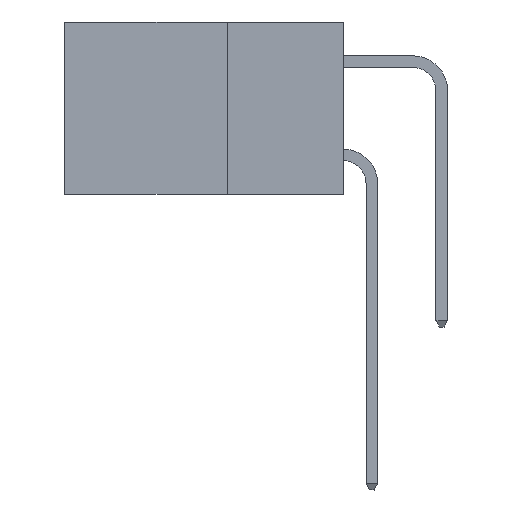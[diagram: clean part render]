
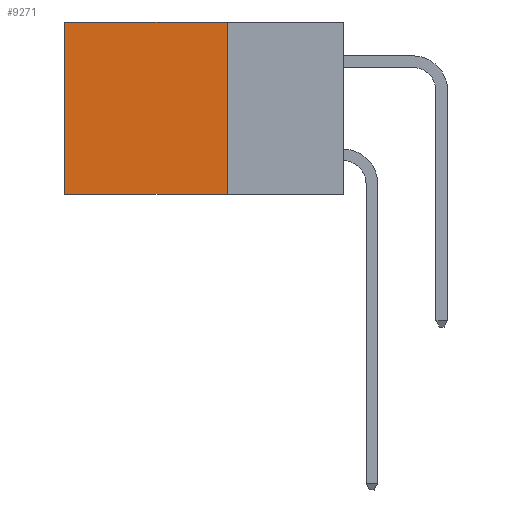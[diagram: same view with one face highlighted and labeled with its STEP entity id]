
A CAD part, left-side view. The second image highlights one B-rep face of the part: STEP entity #9271.
In plain terms, the highlighted planar face has unit normal (-1, 0, 0).
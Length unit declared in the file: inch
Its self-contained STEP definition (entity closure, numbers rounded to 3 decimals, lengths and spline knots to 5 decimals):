
#986 = FACE_OUTER_BOUND ( 'NONE', #16555, .T. ) ;
#1271 = CARTESIAN_POINT ( 'NONE',  ( 0.298, 0.25, -0.37 ) ) ;
#1565 = EDGE_CURVE ( 'NONE', #10299, #5157, #3699, .T. ) ;
#3554 = ORIENTED_EDGE ( 'NONE', *, *, #6476, .F. ) ;
#3699 = LINE ( 'NONE', #14299, #8437 ) ;
#5137 = EDGE_CURVE ( 'NONE', #11124, #12029, #8122, .T. ) ;
#5157 = VERTEX_POINT ( 'NONE', #9886 ) ;
#5939 = DIRECTION ( 'NONE',  ( 0., 0., -1. ) ) ;
#6021 = LINE ( 'NONE', #1271, #13595 ) ;
#6247 = DIRECTION ( 'NONE',  ( 0., 1., 0. ) ) ;
#6289 = VECTOR ( 'NONE', #13048, 39.37008 ) ;
#6476 = EDGE_CURVE ( 'NONE', #12029, #5157, #6021, .T. ) ;
#8122 = LINE ( 'NONE', #13840, #12003 ) ;
#8437 = VECTOR ( 'NONE', #16834, 39.37008 ) ;
#9271 = ADVANCED_FACE ( 'NONE', ( #986 ), #14039, .F. ) ;
#9448 = EDGE_CURVE ( 'NONE', #11124, #10299, #10170, .T. ) ;
#9886 = CARTESIAN_POINT ( 'NONE',  ( 0.298, 0.6, -0.37 ) ) ;
#10089 = CARTESIAN_POINT ( 'NONE',  ( 0.298, 0.25, 0. ) ) ;
#10170 = LINE ( 'NONE', #12938, #6289 ) ;
#10246 = DIRECTION ( 'NONE',  ( 0., 0., -1. ) ) ;
#10299 = VERTEX_POINT ( 'NONE', #11484 ) ;
#10909 = CARTESIAN_POINT ( 'NONE',  ( 0.298, 0.25, -0.37 ) ) ;
#11057 = CARTESIAN_POINT ( 'NONE',  ( 0.298, 0.25, 0. ) ) ;
#11124 = VERTEX_POINT ( 'NONE', #11057 ) ;
#11484 = CARTESIAN_POINT ( 'NONE',  ( 0.298, 0.6, 0. ) ) ;
#11871 = AXIS2_PLACEMENT_3D ( 'NONE', #10089, #13986, #10246 ) ;
#12003 = VECTOR ( 'NONE', #5939, 39.37008 ) ;
#12029 = VERTEX_POINT ( 'NONE', #10909 ) ;
#12938 = CARTESIAN_POINT ( 'NONE',  ( 0.298, 0.25, 0. ) ) ;
#13048 = DIRECTION ( 'NONE',  ( 0., 1., 0. ) ) ;
#13595 = VECTOR ( 'NONE', #6247, 39.37008 ) ;
#13840 = CARTESIAN_POINT ( 'NONE',  ( 0.298, 0.25, 0. ) ) ;
#13986 = DIRECTION ( 'NONE',  ( 1., 0., 0. ) ) ;
#14003 = ORIENTED_EDGE ( 'NONE', *, *, #9448, .T. ) ;
#14039 = PLANE ( 'NONE',  #11871 ) ;
#14299 = CARTESIAN_POINT ( 'NONE',  ( 0.298, 0.6, 0. ) ) ;
#14894 = ORIENTED_EDGE ( 'NONE', *, *, #1565, .T. ) ;
#16004 = ORIENTED_EDGE ( 'NONE', *, *, #5137, .F. ) ;
#16555 = EDGE_LOOP ( 'NONE', ( #14894, #3554, #16004, #14003 ) ) ;
#16834 = DIRECTION ( 'NONE',  ( 0., 0., -1. ) ) ;
